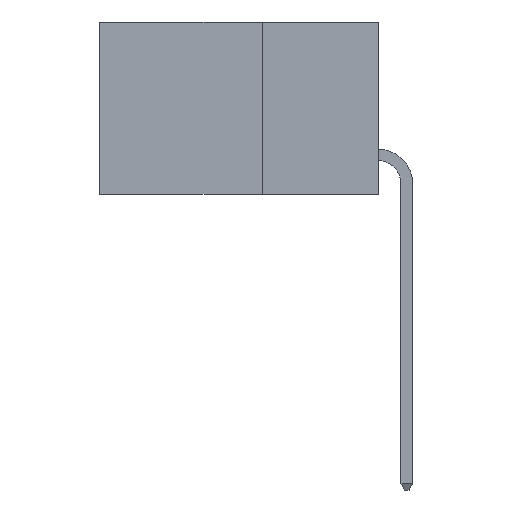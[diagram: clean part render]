
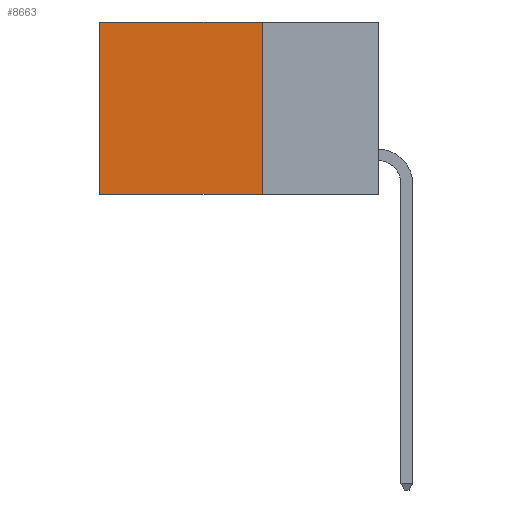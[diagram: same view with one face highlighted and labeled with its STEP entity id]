
A CAD part, left-side view. The second image highlights one B-rep face of the part: STEP entity #8663.
In plain terms, the highlighted planar face has unit normal (-1, 0, 0).
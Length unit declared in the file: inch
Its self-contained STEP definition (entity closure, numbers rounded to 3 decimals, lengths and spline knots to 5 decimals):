
#44 = LINE ( 'NONE', #13038, #10608 ) ;
#89 = ORIENTED_EDGE ( 'NONE', *, *, #3535, .F. ) ;
#293 = LINE ( 'NONE', #8967, #7219 ) ;
#387 = LINE ( 'NONE', #4665, #1250 ) ;
#456 = DIRECTION ( 'NONE',  ( 0., 0., -1. ) ) ;
#508 = PLANE ( 'NONE',  #2619 ) ;
#1250 = VECTOR ( 'NONE', #3572, 39.37008 ) ;
#2619 = AXIS2_PLACEMENT_3D ( 'NONE', #8220, #2885, #456 ) ;
#2885 = DIRECTION ( 'NONE',  ( 1., 0., 0. ) ) ;
#3535 = EDGE_CURVE ( 'NONE', #10246, #13079, #387, .T. ) ;
#3572 = DIRECTION ( 'NONE',  ( 0., 1., 0. ) ) ;
#3863 = CARTESIAN_POINT ( 'NONE',  ( 0.2615, 0.25, -0.37 ) ) ;
#4319 = VECTOR ( 'NONE', #11587, 39.37008 ) ;
#4665 = CARTESIAN_POINT ( 'NONE',  ( 0.2615, 0.25, -0.37 ) ) ;
#6108 = CARTESIAN_POINT ( 'NONE',  ( 0.2615, 0.25, 0. ) ) ;
#6624 = EDGE_CURVE ( 'NONE', #7399, #10246, #293, .T. ) ;
#7219 = VECTOR ( 'NONE', #9207, 39.37008 ) ;
#7268 = EDGE_CURVE ( 'NONE', #12536, #13079, #44, .T. ) ;
#7399 = VERTEX_POINT ( 'NONE', #11761 ) ;
#8220 = CARTESIAN_POINT ( 'NONE',  ( 0.2615, 0.25, -0.37 ) ) ;
#8663 = ADVANCED_FACE ( 'NONE', ( #16672 ), #508, .F. ) ;
#8666 = CARTESIAN_POINT ( 'NONE',  ( 0.2615, 0.6, -0.37 ) ) ;
#8805 = CARTESIAN_POINT ( 'NONE',  ( 0.2615, 0.6, 0. ) ) ;
#8967 = CARTESIAN_POINT ( 'NONE',  ( 0.2615, 0.25, -0.37 ) ) ;
#9207 = DIRECTION ( 'NONE',  ( 0., 0., -1. ) ) ;
#9540 = ORIENTED_EDGE ( 'NONE', *, *, #6624, .F. ) ;
#10246 = VERTEX_POINT ( 'NONE', #3863 ) ;
#10608 = VECTOR ( 'NONE', #12993, 39.37008 ) ;
#10668 = EDGE_CURVE ( 'NONE', #7399, #12536, #15178, .T. ) ;
#11587 = DIRECTION ( 'NONE',  ( 0., 1., 0. ) ) ;
#11656 = ORIENTED_EDGE ( 'NONE', *, *, #10668, .T. ) ;
#11761 = CARTESIAN_POINT ( 'NONE',  ( 0.2615, 0.25, 0. ) ) ;
#12536 = VERTEX_POINT ( 'NONE', #8805 ) ;
#12993 = DIRECTION ( 'NONE',  ( 0., 0., -1. ) ) ;
#13038 = CARTESIAN_POINT ( 'NONE',  ( 0.2615, 0.6, -0.37 ) ) ;
#13079 = VERTEX_POINT ( 'NONE', #8666 ) ;
#13599 = ORIENTED_EDGE ( 'NONE', *, *, #7268, .T. ) ;
#15178 = LINE ( 'NONE', #6108, #4319 ) ;
#15760 = EDGE_LOOP ( 'NONE', ( #13599, #89, #9540, #11656 ) ) ;
#16672 = FACE_OUTER_BOUND ( 'NONE', #15760, .T. ) ;
